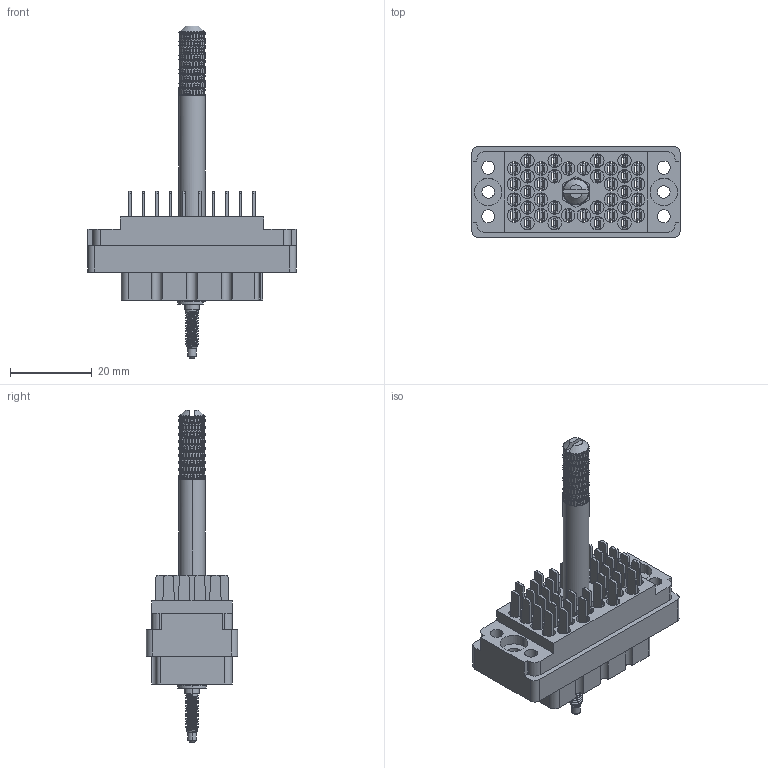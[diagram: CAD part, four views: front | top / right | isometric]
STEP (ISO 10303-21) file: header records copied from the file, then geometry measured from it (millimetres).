
FILE_DESCRIPTION (( 'STEP AP203' ), '1' );
FILE_NAME ('516-038-501-405.STEP', '2020-09-08T15:05:55', ( '' ), ( '' ), 'SwSTEP 2.0', 'SolidWorks 2020', '' );
FILE_SCHEMA (( 'CONFIG_CONTROL_DESIGN' ));
Length unit declared in the file: inch
Products named in the file (8): 516-251-035-100; 516-038-501-405; 516-250-038-111; 516-253-138-107; 516 Part Receptacle_038; Actuating Screw Assy 038-056; 516-292-001_501 Contact; 516-253-035-100
Assembly tree (46 placements, depth 3):
  516-038-501-405
    516 Part Receptacle_038
    516-292-001_501 Contact  x39
    Actuating Screw Assy 038-056
      516-251-035-100
      516-253-035-100  x2
      516-253-138-107
      516-250-038-111
Bounding box: 50.8 x 22.25 x 81.03 mm (x, y, z)
Volume: 14204.2 mm3; surface area: 23767.2 mm2
Topology: 45 solids, 45 shells, 5125 faces, 13808 edges, 8792 vertices
Faces by surface type: plane 2312, cylinder 1553, bspline 1240, cone 20
Entity records: 101583 total; most frequent: CARTESIAN_POINT 54313, ORIENTED_EDGE 11784, DIRECTION 6976, EDGE_CURVE 5892, VERTEX_POINT 3540, EDGE_LOOP 2498, FACE_OUTER_BOUND 2383, ADVANCED_FACE 2383
